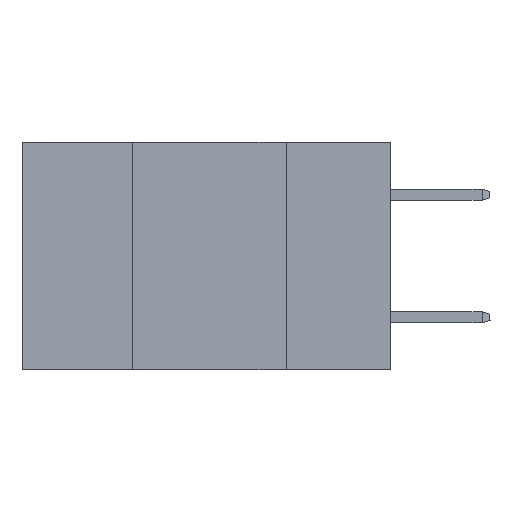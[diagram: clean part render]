
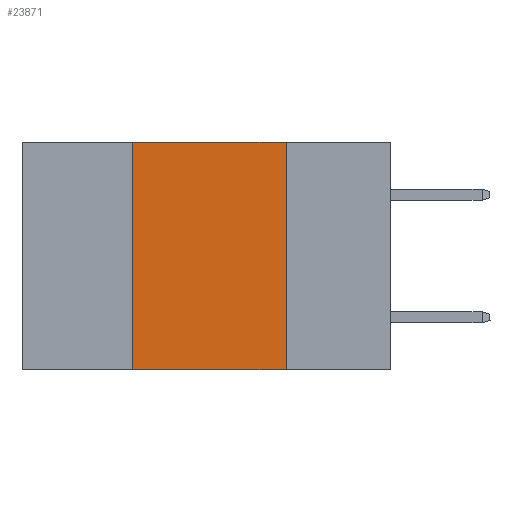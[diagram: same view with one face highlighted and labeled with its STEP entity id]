
A CAD part, left-side view. The second image highlights one B-rep face of the part: STEP entity #23871.
In plain terms, the highlighted planar face has unit normal (-1, 0, 0).
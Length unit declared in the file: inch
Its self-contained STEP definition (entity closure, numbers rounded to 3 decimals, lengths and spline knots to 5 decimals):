
#163 = VERTEX_POINT ( 'NONE', #17075 ) ;
#875 = EDGE_LOOP ( 'NONE', ( #33782, #7970, #35067, #4624 ) ) ;
#949 = CARTESIAN_POINT ( 'NONE',  ( 0., 0.17, -0.37 ) ) ;
#1097 = VECTOR ( 'NONE', #21169, 39.37008 ) ;
#1780 = VECTOR ( 'NONE', #4657, 39.37008 ) ;
#2237 = CARTESIAN_POINT ( 'NONE',  ( 0., 0.6, 0. ) ) ;
#3813 = VECTOR ( 'NONE', #27716, 39.37008 ) ;
#4624 = ORIENTED_EDGE ( 'NONE', *, *, #15528, .T. ) ;
#4657 = DIRECTION ( 'NONE',  ( 0., 0., 1. ) ) ;
#6153 = EDGE_CURVE ( 'NONE', #14071, #14708, #31317, .T. ) ;
#6823 = VERTEX_POINT ( 'NONE', #949 ) ;
#7970 = ORIENTED_EDGE ( 'NONE', *, *, #6153, .F. ) ;
#9436 = CARTESIAN_POINT ( 'NONE',  ( 0., 0.17, 0. ) ) ;
#10988 = PLANE ( 'NONE',  #30158 ) ;
#11384 = DIRECTION ( 'NONE',  ( 1., 0., 0. ) ) ;
#13242 = EDGE_CURVE ( 'NONE', #14708, #6823, #30970, .T. ) ;
#13398 = CARTESIAN_POINT ( 'NONE',  ( 0., 0.42, 0. ) ) ;
#14071 = VERTEX_POINT ( 'NONE', #27032 ) ;
#14708 = VERTEX_POINT ( 'NONE', #21622 ) ;
#15528 = EDGE_CURVE ( 'NONE', #163, #6823, #20714, .T. ) ;
#16305 = VECTOR ( 'NONE', #36934, 39.37008 ) ;
#17075 = CARTESIAN_POINT ( 'NONE',  ( 0., 0.42, -0.37 ) ) ;
#20714 = LINE ( 'NONE', #39753, #16305 ) ;
#21169 = DIRECTION ( 'NONE',  ( 0., -1., 0. ) ) ;
#21622 = CARTESIAN_POINT ( 'NONE',  ( 0., 0.17, 0. ) ) ;
#23155 = LINE ( 'NONE', #13398, #1780 ) ;
#23871 = ADVANCED_FACE ( 'NONE', ( #38203 ), #10988, .F. ) ;
#26434 = DIRECTION ( 'NONE',  ( 0., 0., -1. ) ) ;
#27032 = CARTESIAN_POINT ( 'NONE',  ( 0., 0.42, 0. ) ) ;
#27716 = DIRECTION ( 'NONE',  ( 0., 0., -1. ) ) ;
#28739 = EDGE_CURVE ( 'NONE', #163, #14071, #23155, .T. ) ;
#30158 = AXIS2_PLACEMENT_3D ( 'NONE', #2237, #11384, #26434 ) ;
#30517 = CARTESIAN_POINT ( 'NONE',  ( 0., 0.6, 0. ) ) ;
#30970 = LINE ( 'NONE', #9436, #3813 ) ;
#31317 = LINE ( 'NONE', #30517, #1097 ) ;
#33782 = ORIENTED_EDGE ( 'NONE', *, *, #13242, .F. ) ;
#35067 = ORIENTED_EDGE ( 'NONE', *, *, #28739, .F. ) ;
#36934 = DIRECTION ( 'NONE',  ( 0., -1., 0. ) ) ;
#38203 = FACE_OUTER_BOUND ( 'NONE', #875, .T. ) ;
#39753 = CARTESIAN_POINT ( 'NONE',  ( 0., 0.6, -0.37 ) ) ;
